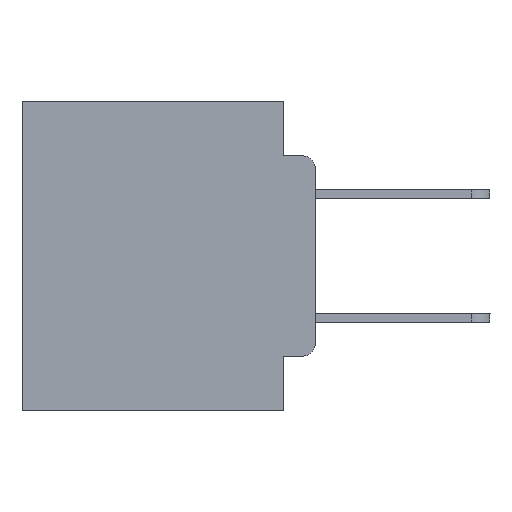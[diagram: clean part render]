
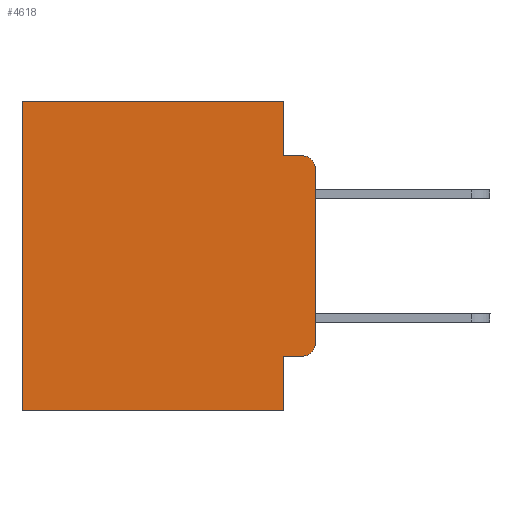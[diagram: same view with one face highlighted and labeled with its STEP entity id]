
A CAD part, left-side view. The second image highlights one B-rep face of the part: STEP entity #4618.
In plain terms, the highlighted planar face has unit normal (-1, 0, 0).
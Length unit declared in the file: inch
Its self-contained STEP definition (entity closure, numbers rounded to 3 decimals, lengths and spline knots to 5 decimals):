
#360 = ORIENTED_EDGE ( 'NONE', *, *, #23469, .F. ) ;
#673 = CARTESIAN_POINT ( 'NONE',  ( 0.298, 0.02, -0.1085 ) ) ;
#1038 = FACE_OUTER_BOUND ( 'NONE', #18245, .T. ) ;
#1341 = DIRECTION ( 'NONE',  ( 1., 0., 0. ) ) ;
#1787 = ORIENTED_EDGE ( 'NONE', *, *, #17757, .F. ) ;
#1985 = ORIENTED_EDGE ( 'NONE', *, *, #13458, .T. ) ;
#2032 = VECTOR ( 'NONE', #5464, 39.37008 ) ;
#2065 = CARTESIAN_POINT ( 'NONE',  ( 0.298, 0.473, 0. ) ) ;
#2332 = CARTESIAN_POINT ( 'NONE',  ( 0.298, 0.051, -0.4115 ) ) ;
#2427 = CARTESIAN_POINT ( 'NONE',  ( 0.298, 0.02, -0.4115 ) ) ;
#4157 = CARTESIAN_POINT ( 'NONE',  ( 0.298, 0.051, -0.0885 ) ) ;
#4618 = ADVANCED_FACE ( 'NONE', ( #1038 ), #19588, .F. ) ;
#4835 = VECTOR ( 'NONE', #10585, 39.37008 ) ;
#4945 = DIRECTION ( 'NONE',  ( 0., 0., -1. ) ) ;
#5322 = DIRECTION ( 'NONE',  ( 0., 1., 0. ) ) ;
#5324 = DIRECTION ( 'NONE',  ( 0., 0., -1. ) ) ;
#5464 = DIRECTION ( 'NONE',  ( 0., 0., -1. ) ) ;
#5528 = CARTESIAN_POINT ( 'NONE',  ( 0.298, 0.473, 0. ) ) ;
#5860 = ORIENTED_EDGE ( 'NONE', *, *, #17488, .F. ) ;
#7022 = LINE ( 'NONE', #18843, #18135 ) ;
#7881 = CIRCLE ( 'NONE', #15169, 0.02 ) ;
#8180 = EDGE_CURVE ( 'NONE', #24122, #10841, #11959, .T. ) ;
#8550 = VERTEX_POINT ( 'NONE', #12841 ) ;
#8673 = AXIS2_PLACEMENT_3D ( 'NONE', #17602, #1341, #13499 ) ;
#9017 = VECTOR ( 'NONE', #20900, 39.37008 ) ;
#9131 = ORIENTED_EDGE ( 'NONE', *, *, #8180, .T. ) ;
#10414 = EDGE_CURVE ( 'NONE', #17536, #24122, #17566, .T. ) ;
#10585 = DIRECTION ( 'NONE',  ( 0., 0., -1. ) ) ;
#10841 = VERTEX_POINT ( 'NONE', #17515 ) ;
#10884 = LINE ( 'NONE', #2332, #9017 ) ;
#11012 = EDGE_CURVE ( 'NONE', #22285, #18284, #13399, .T. ) ;
#11062 = CARTESIAN_POINT ( 'NONE',  ( 0.298, 0., 0. ) ) ;
#11507 = VERTEX_POINT ( 'NONE', #25873 ) ;
#11852 = DIRECTION ( 'NONE',  ( 0., 0., -1. ) ) ;
#11959 = LINE ( 'NONE', #2065, #24078 ) ;
#12841 = CARTESIAN_POINT ( 'NONE',  ( 0.298, 0.02, -0.0885 ) ) ;
#13399 = LINE ( 'NONE', #26238, #4835 ) ;
#13423 = EDGE_CURVE ( 'NONE', #18284, #10841, #13672, .T. ) ;
#13458 = EDGE_CURVE ( 'NONE', #25939, #11507, #25415, .T. ) ;
#13499 = DIRECTION ( 'NONE',  ( 0., 0., -1. ) ) ;
#13672 = LINE ( 'NONE', #17411, #22876 ) ;
#13823 = CARTESIAN_POINT ( 'NONE',  ( 0.298, 0.02, -0.3915 ) ) ;
#14550 = CARTESIAN_POINT ( 'NONE',  ( 0.298, 0.051, -0.5 ) ) ;
#14947 = CARTESIAN_POINT ( 'NONE',  ( 0.298, 0., -0.1085 ) ) ;
#15169 = AXIS2_PLACEMENT_3D ( 'NONE', #673, #24953, #4945 ) ;
#15347 = VECTOR ( 'NONE', #23455, 39.37008 ) ;
#15531 = DIRECTION ( 'NONE',  ( 0., 0., -1. ) ) ;
#15644 = ORIENTED_EDGE ( 'NONE', *, *, #24435, .T. ) ;
#15710 = DIRECTION ( 'NONE',  ( -1., 0., 0. ) ) ;
#16758 = ORIENTED_EDGE ( 'NONE', *, *, #11012, .F. ) ;
#16830 = ORIENTED_EDGE ( 'NONE', *, *, #19796, .T. ) ;
#17029 = DIRECTION ( 'NONE',  ( 0., -1., 0. ) ) ;
#17411 = CARTESIAN_POINT ( 'NONE',  ( 0.298, 0., -0.5 ) ) ;
#17418 = ORIENTED_EDGE ( 'NONE', *, *, #10414, .T. ) ;
#17488 = EDGE_CURVE ( 'NONE', #17536, #20099, #21998, .T. ) ;
#17515 = CARTESIAN_POINT ( 'NONE',  ( 0.298, 0.473, -0.5 ) ) ;
#17536 = VERTEX_POINT ( 'NONE', #18844 ) ;
#17566 = LINE ( 'NONE', #11062, #15347 ) ;
#17602 = CARTESIAN_POINT ( 'NONE',  ( 0.298, 0., 0. ) ) ;
#17757 = EDGE_CURVE ( 'NONE', #20099, #8550, #7022, .T. ) ;
#18135 = VECTOR ( 'NONE', #17029, 39.37008 ) ;
#18245 = EDGE_LOOP ( 'NONE', ( #360, #16830, #1787, #5860, #17418, #9131, #22142, #16758, #15644, #1985 ) ) ;
#18284 = VERTEX_POINT ( 'NONE', #14550 ) ;
#18843 = CARTESIAN_POINT ( 'NONE',  ( 0.298, 0.051, -0.0885 ) ) ;
#18844 = CARTESIAN_POINT ( 'NONE',  ( 0.298, 0.051, 0. ) ) ;
#19588 = PLANE ( 'NONE',  #8673 ) ;
#19796 = EDGE_CURVE ( 'NONE', #25349, #8550, #7881, .T. ) ;
#20099 = VERTEX_POINT ( 'NONE', #4157 ) ;
#20900 = DIRECTION ( 'NONE',  ( 0., -1., 0. ) ) ;
#21998 = LINE ( 'NONE', #25849, #25807 ) ;
#22142 = ORIENTED_EDGE ( 'NONE', *, *, #13423, .F. ) ;
#22151 = CARTESIAN_POINT ( 'NONE',  ( 0.298, 0.051, -0.4115 ) ) ;
#22285 = VERTEX_POINT ( 'NONE', #22151 ) ;
#22876 = VECTOR ( 'NONE', #5322, 39.37008 ) ;
#22960 = AXIS2_PLACEMENT_3D ( 'NONE', #13823, #15710, #15531 ) ;
#23314 = LINE ( 'NONE', #26110, #2032 ) ;
#23455 = DIRECTION ( 'NONE',  ( 0., 1., 0. ) ) ;
#23469 = EDGE_CURVE ( 'NONE', #25349, #11507, #23314, .T. ) ;
#24078 = VECTOR ( 'NONE', #5324, 39.37008 ) ;
#24122 = VERTEX_POINT ( 'NONE', #5528 ) ;
#24435 = EDGE_CURVE ( 'NONE', #22285, #25939, #10884, .T. ) ;
#24953 = DIRECTION ( 'NONE',  ( -1., 0., 0. ) ) ;
#25349 = VERTEX_POINT ( 'NONE', #14947 ) ;
#25415 = CIRCLE ( 'NONE', #22960, 0.02 ) ;
#25807 = VECTOR ( 'NONE', #11852, 39.37008 ) ;
#25849 = CARTESIAN_POINT ( 'NONE',  ( 0.298, 0.051, 0. ) ) ;
#25873 = CARTESIAN_POINT ( 'NONE',  ( 0.298, 0., -0.3915 ) ) ;
#25939 = VERTEX_POINT ( 'NONE', #2427 ) ;
#26110 = CARTESIAN_POINT ( 'NONE',  ( 0.298, 0., 0. ) ) ;
#26238 = CARTESIAN_POINT ( 'NONE',  ( 0.298, 0.051, 0. ) ) ;
